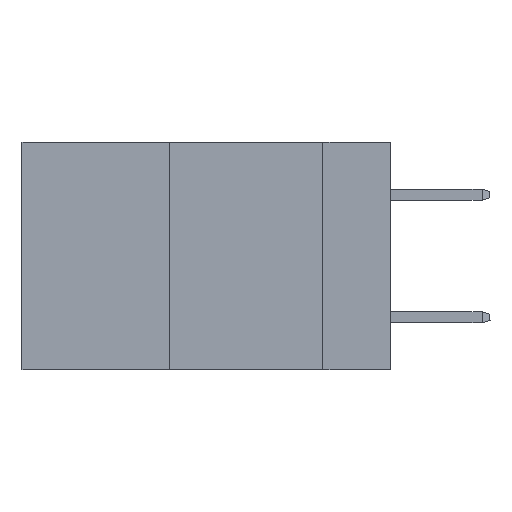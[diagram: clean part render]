
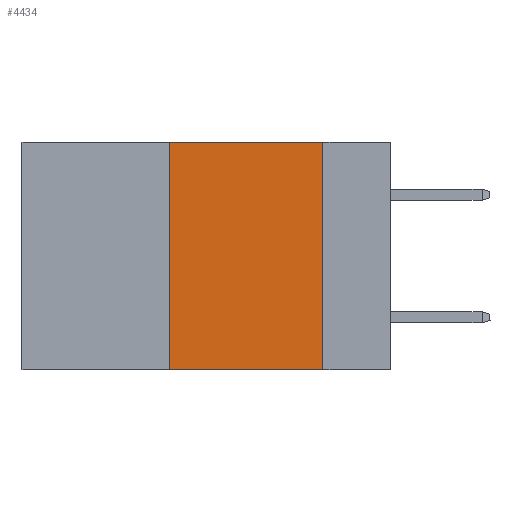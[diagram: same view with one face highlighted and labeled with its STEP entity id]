
A CAD part, left-side view. The second image highlights one B-rep face of the part: STEP entity #4434.
In plain terms, the highlighted planar face has unit normal (-1, 0, 0).
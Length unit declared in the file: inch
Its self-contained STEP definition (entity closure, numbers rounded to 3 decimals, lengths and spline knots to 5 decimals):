
#255 = CARTESIAN_POINT ( 'NONE',  ( 0., 0.11, 0. ) ) ;
#292 = EDGE_CURVE ( 'NONE', #10560, #9604, #3147, .T. ) ;
#347 = VECTOR ( 'NONE', #11560, 39.37008 ) ;
#543 = VERTEX_POINT ( 'NONE', #4145 ) ;
#1489 = EDGE_CURVE ( 'NONE', #543, #9604, #2219, .T. ) ;
#2020 = EDGE_CURVE ( 'NONE', #7141, #543, #6007, .T. ) ;
#2219 = LINE ( 'NONE', #255, #3745 ) ;
#2531 = EDGE_LOOP ( 'NONE', ( #8426, #10219, #3063, #7217 ) ) ;
#2571 = FACE_OUTER_BOUND ( 'NONE', #2531, .T. ) ;
#2624 = CARTESIAN_POINT ( 'NONE',  ( 0., 0.6, -0.37 ) ) ;
#3063 = ORIENTED_EDGE ( 'NONE', *, *, #4152, .F. ) ;
#3147 = LINE ( 'NONE', #2624, #347 ) ;
#3241 = CARTESIAN_POINT ( 'NONE',  ( 0., 0.11, -0.37 ) ) ;
#3714 = DIRECTION ( 'NONE',  ( 0., 0., -1. ) ) ;
#3745 = VECTOR ( 'NONE', #6835, 39.37008 ) ;
#4145 = CARTESIAN_POINT ( 'NONE',  ( 0., 0.11, 0. ) ) ;
#4152 = EDGE_CURVE ( 'NONE', #10560, #7141, #7484, .T. ) ;
#4434 = ADVANCED_FACE ( 'NONE', ( #2571 ), #12131, .F. ) ;
#6007 = LINE ( 'NONE', #9698, #8302 ) ;
#6189 = DIRECTION ( 'NONE',  ( 0., -1., 0. ) ) ;
#6835 = DIRECTION ( 'NONE',  ( 0., 0., -1. ) ) ;
#6909 = AXIS2_PLACEMENT_3D ( 'NONE', #8035, #11841, #3714 ) ;
#7141 = VERTEX_POINT ( 'NONE', #8397 ) ;
#7217 = ORIENTED_EDGE ( 'NONE', *, *, #292, .T. ) ;
#7484 = LINE ( 'NONE', #11167, #10150 ) ;
#8035 = CARTESIAN_POINT ( 'NONE',  ( 0., 0.6, 0. ) ) ;
#8302 = VECTOR ( 'NONE', #6189, 39.37008 ) ;
#8397 = CARTESIAN_POINT ( 'NONE',  ( 0., 0.36, 0. ) ) ;
#8407 = CARTESIAN_POINT ( 'NONE',  ( 0., 0.36, -0.37 ) ) ;
#8426 = ORIENTED_EDGE ( 'NONE', *, *, #1489, .F. ) ;
#9276 = DIRECTION ( 'NONE',  ( 0., 0., 1. ) ) ;
#9604 = VERTEX_POINT ( 'NONE', #3241 ) ;
#9698 = CARTESIAN_POINT ( 'NONE',  ( 0., 0.6, 0. ) ) ;
#10150 = VECTOR ( 'NONE', #9276, 39.37008 ) ;
#10219 = ORIENTED_EDGE ( 'NONE', *, *, #2020, .F. ) ;
#10560 = VERTEX_POINT ( 'NONE', #8407 ) ;
#11167 = CARTESIAN_POINT ( 'NONE',  ( 0., 0.36, 0. ) ) ;
#11560 = DIRECTION ( 'NONE',  ( 0., -1., 0. ) ) ;
#11841 = DIRECTION ( 'NONE',  ( 1., 0., 0. ) ) ;
#12131 = PLANE ( 'NONE',  #6909 ) ;
